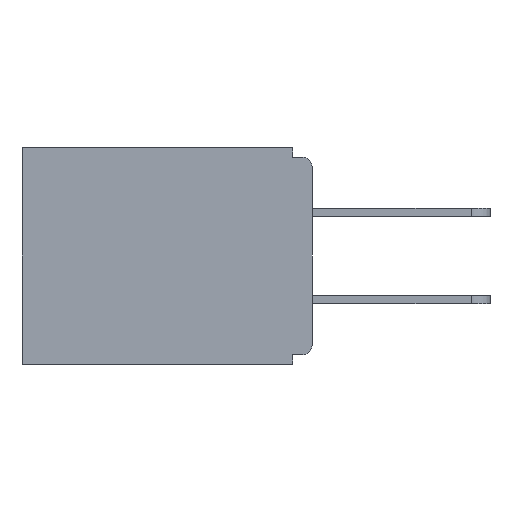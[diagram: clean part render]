
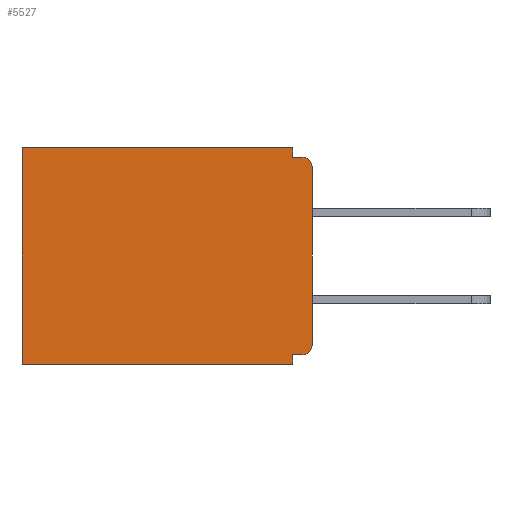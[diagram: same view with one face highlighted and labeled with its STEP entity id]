
A CAD part, left-side view. The second image highlights one B-rep face of the part: STEP entity #5527.
In plain terms, the highlighted planar face has unit normal (-1, 0, 0).
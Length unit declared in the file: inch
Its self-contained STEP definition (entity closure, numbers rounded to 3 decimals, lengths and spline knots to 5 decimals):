
#186 = CARTESIAN_POINT ( 'NONE',  ( 0.298, 0.031, -0.343 ) ) ;
#228 = VECTOR ( 'NONE', #4680, 39.37008 ) ;
#256 = VERTEX_POINT ( 'NONE', #11042 ) ;
#363 = LINE ( 'NONE', #2710, #228 ) ;
#385 = EDGE_CURVE ( 'NONE', #4283, #12526, #6607, .T. ) ;
#410 = EDGE_CURVE ( 'NONE', #2976, #256, #1720, .T. ) ;
#529 = ORIENTED_EDGE ( 'NONE', *, *, #385, .F. ) ;
#785 = VECTOR ( 'NONE', #4152, 39.37008 ) ;
#1202 = CARTESIAN_POINT ( 'NONE',  ( 0.298, 0.031, -0.343 ) ) ;
#1569 = VERTEX_POINT ( 'NONE', #4419 ) ;
#1594 = CARTESIAN_POINT ( 'NONE',  ( 0.298, 0.46, -0.343 ) ) ;
#1630 = CARTESIAN_POINT ( 'NONE',  ( 0.298, 0., -0.03 ) ) ;
#1720 = LINE ( 'NONE', #7551, #7352 ) ;
#2067 = ORIENTED_EDGE ( 'NONE', *, *, #410, .F. ) ;
#2138 = LINE ( 'NONE', #9085, #2445 ) ;
#2249 = ORIENTED_EDGE ( 'NONE', *, *, #9962, .T. ) ;
#2301 = AXIS2_PLACEMENT_3D ( 'NONE', #5526, #3653, #8369 ) ;
#2366 = CARTESIAN_POINT ( 'NONE',  ( 0.298, 0.015, -0.328 ) ) ;
#2445 = VECTOR ( 'NONE', #3278, 39.37008 ) ;
#2509 = EDGE_CURVE ( 'NONE', #11962, #11312, #2530, .T. ) ;
#2530 = LINE ( 'NONE', #5929, #9240 ) ;
#2710 = CARTESIAN_POINT ( 'NONE',  ( 0.298, 0., -0.343 ) ) ;
#2715 = CIRCLE ( 'NONE', #2301, 0.015 ) ;
#2898 = ORIENTED_EDGE ( 'NONE', *, *, #8842, .T. ) ;
#2947 = DIRECTION ( 'NONE',  ( 0., -1., 0. ) ) ;
#2976 = VERTEX_POINT ( 'NONE', #1630 ) ;
#3116 = DIRECTION ( 'NONE',  ( 0., 0., -1. ) ) ;
#3170 = VECTOR ( 'NONE', #10478, 39.37008 ) ;
#3278 = DIRECTION ( 'NONE',  ( 0., 0., -1. ) ) ;
#3378 = VERTEX_POINT ( 'NONE', #1202 ) ;
#3583 = EDGE_LOOP ( 'NONE', ( #2249, #5073, #10915, #10820, #2898, #10057, #8966, #529, #10034, #2067 ) ) ;
#3653 = DIRECTION ( 'NONE',  ( -1., 0., 0. ) ) ;
#4021 = VERTEX_POINT ( 'NONE', #1594 ) ;
#4061 = DIRECTION ( 'NONE',  ( -1., 0., 0. ) ) ;
#4152 = DIRECTION ( 'NONE',  ( 0., 1., 0. ) ) ;
#4283 = VERTEX_POINT ( 'NONE', #2366 ) ;
#4356 = AXIS2_PLACEMENT_3D ( 'NONE', #9871, #4061, #5043 ) ;
#4419 = CARTESIAN_POINT ( 'NONE',  ( 0.298, 0.46, 0. ) ) ;
#4425 = LINE ( 'NONE', #186, #9423 ) ;
#4680 = DIRECTION ( 'NONE',  ( 0., 1., 0. ) ) ;
#4877 = EDGE_CURVE ( 'NONE', #3378, #4021, #363, .T. ) ;
#5043 = DIRECTION ( 'NONE',  ( 0., 0., -1. ) ) ;
#5063 = CARTESIAN_POINT ( 'NONE',  ( 0.298, 0.031, -0.328 ) ) ;
#5073 = ORIENTED_EDGE ( 'NONE', *, *, #2509, .F. ) ;
#5411 = CARTESIAN_POINT ( 'NONE',  ( 0.298, 0., -0.328 ) ) ;
#5450 = LINE ( 'NONE', #11451, #3170 ) ;
#5460 = DIRECTION ( 'NONE',  ( 0., 1., 0. ) ) ;
#5486 = CARTESIAN_POINT ( 'NONE',  ( 0.298, 0.015, -0.015 ) ) ;
#5526 = CARTESIAN_POINT ( 'NONE',  ( 0.298, 0.015, -0.03 ) ) ;
#5527 = ADVANCED_FACE ( 'NONE', ( #6144 ), #8202, .F. ) ;
#5929 = CARTESIAN_POINT ( 'NONE',  ( 0.298, 0., -0.015 ) ) ;
#6144 = FACE_OUTER_BOUND ( 'NONE', #3583, .T. ) ;
#6251 = DIRECTION ( 'NONE',  ( 1., 0., 0. ) ) ;
#6449 = CARTESIAN_POINT ( 'NONE',  ( 0.298, 0., 0. ) ) ;
#6480 = EDGE_CURVE ( 'NONE', #7767, #1569, #7927, .T. ) ;
#6607 = LINE ( 'NONE', #5411, #8725 ) ;
#6921 = EDGE_CURVE ( 'NONE', #7767, #11962, #4425, .T. ) ;
#7352 = VECTOR ( 'NONE', #7418, 39.37008 ) ;
#7418 = DIRECTION ( 'NONE',  ( 0., 0., -1. ) ) ;
#7551 = CARTESIAN_POINT ( 'NONE',  ( 0.298, 0., 0. ) ) ;
#7767 = VERTEX_POINT ( 'NONE', #11949 ) ;
#7927 = LINE ( 'NONE', #6449, #785 ) ;
#8202 = PLANE ( 'NONE',  #11039 ) ;
#8319 = EDGE_CURVE ( 'NONE', #4283, #256, #10668, .T. ) ;
#8369 = DIRECTION ( 'NONE',  ( 0., 0., -1. ) ) ;
#8725 = VECTOR ( 'NONE', #5460, 39.37008 ) ;
#8842 = EDGE_CURVE ( 'NONE', #1569, #4021, #2138, .T. ) ;
#8966 = ORIENTED_EDGE ( 'NONE', *, *, #10682, .F. ) ;
#9085 = CARTESIAN_POINT ( 'NONE',  ( 0.298, 0.46, 0. ) ) ;
#9114 = CARTESIAN_POINT ( 'NONE',  ( 0.298, 0.031, -0.015 ) ) ;
#9240 = VECTOR ( 'NONE', #2947, 39.37008 ) ;
#9423 = VECTOR ( 'NONE', #3116, 39.37008 ) ;
#9871 = CARTESIAN_POINT ( 'NONE',  ( 0.298, 0.015, -0.313 ) ) ;
#9962 = EDGE_CURVE ( 'NONE', #2976, #11312, #2715, .T. ) ;
#10034 = ORIENTED_EDGE ( 'NONE', *, *, #8319, .T. ) ;
#10057 = ORIENTED_EDGE ( 'NONE', *, *, #4877, .F. ) ;
#10478 = DIRECTION ( 'NONE',  ( 0., 0., -1. ) ) ;
#10668 = CIRCLE ( 'NONE', #4356, 0.015 ) ;
#10682 = EDGE_CURVE ( 'NONE', #12526, #3378, #5450, .T. ) ;
#10820 = ORIENTED_EDGE ( 'NONE', *, *, #6480, .T. ) ;
#10915 = ORIENTED_EDGE ( 'NONE', *, *, #6921, .F. ) ;
#11039 = AXIS2_PLACEMENT_3D ( 'NONE', #12125, #6251, #11109 ) ;
#11042 = CARTESIAN_POINT ( 'NONE',  ( 0.298, 0., -0.313 ) ) ;
#11109 = DIRECTION ( 'NONE',  ( 0., 0., -1. ) ) ;
#11312 = VERTEX_POINT ( 'NONE', #5486 ) ;
#11451 = CARTESIAN_POINT ( 'NONE',  ( 0.298, 0.031, -0.343 ) ) ;
#11949 = CARTESIAN_POINT ( 'NONE',  ( 0.298, 0.031, 0. ) ) ;
#11962 = VERTEX_POINT ( 'NONE', #9114 ) ;
#12125 = CARTESIAN_POINT ( 'NONE',  ( 0.298, 0., 0. ) ) ;
#12526 = VERTEX_POINT ( 'NONE', #5063 ) ;
